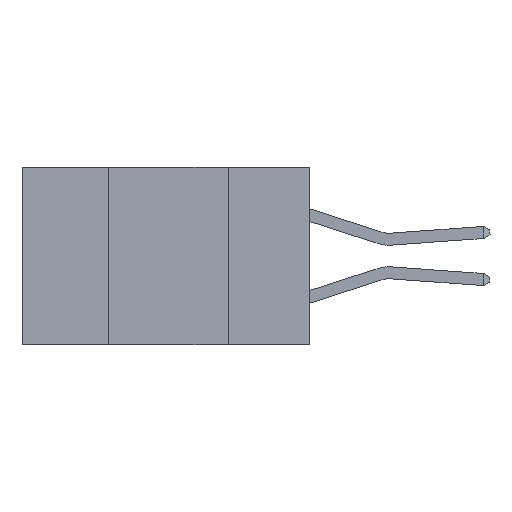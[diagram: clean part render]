
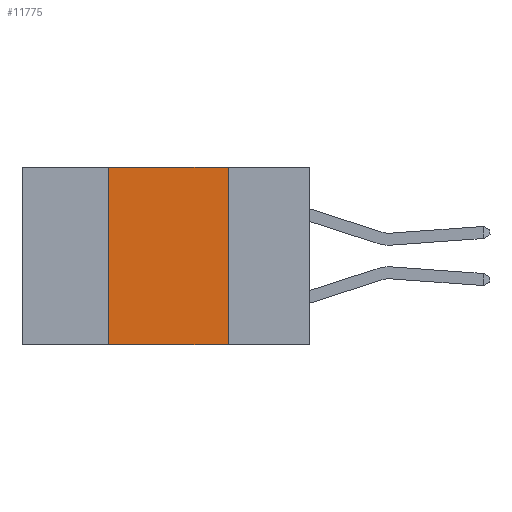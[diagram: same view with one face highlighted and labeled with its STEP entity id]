
A CAD part, left-side view. The second image highlights one B-rep face of the part: STEP entity #11775.
In plain terms, the highlighted planar face has unit normal (-1, 0, 0).
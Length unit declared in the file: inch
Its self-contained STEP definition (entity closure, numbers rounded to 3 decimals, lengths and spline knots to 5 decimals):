
#38 = DIRECTION ( 'NONE',  ( 1., 0., 0. ) ) ;
#1199 = VECTOR ( 'NONE', #7172, 39.37008 ) ;
#1206 = VECTOR ( 'NONE', #1459, 39.37008 ) ;
#1294 = CARTESIAN_POINT ( 'NONE',  ( 0., 0.42, -0.37 ) ) ;
#1459 = DIRECTION ( 'NONE',  ( 0., -1., 0. ) ) ;
#2336 = CARTESIAN_POINT ( 'NONE',  ( 0., 0.17, 0. ) ) ;
#2898 = DIRECTION ( 'NONE',  ( 0., -1., 0. ) ) ;
#3753 = VERTEX_POINT ( 'NONE', #1294 ) ;
#4322 = VERTEX_POINT ( 'NONE', #10105 ) ;
#4729 = LINE ( 'NONE', #11381, #13402 ) ;
#5004 = DIRECTION ( 'NONE',  ( 0., 0., 1. ) ) ;
#5366 = ORIENTED_EDGE ( 'NONE', *, *, #13936, .T. ) ;
#6146 = CARTESIAN_POINT ( 'NONE',  ( 0., 0.42, 0. ) ) ;
#6236 = ORIENTED_EDGE ( 'NONE', *, *, #10648, .F. ) ;
#6549 = FACE_OUTER_BOUND ( 'NONE', #13334, .T. ) ;
#6702 = VECTOR ( 'NONE', #5004, 39.37008 ) ;
#7078 = LINE ( 'NONE', #13237, #6702 ) ;
#7113 = VERTEX_POINT ( 'NONE', #12427 ) ;
#7172 = DIRECTION ( 'NONE',  ( 0., 0., -1. ) ) ;
#7542 = ORIENTED_EDGE ( 'NONE', *, *, #14920, .F. ) ;
#7677 = LINE ( 'NONE', #2336, #1199 ) ;
#8503 = CARTESIAN_POINT ( 'NONE',  ( 0., 0.6, 0. ) ) ;
#8557 = DIRECTION ( 'NONE',  ( 0., 0., -1. ) ) ;
#8748 = CARTESIAN_POINT ( 'NONE',  ( 0., 0.6, -0.37 ) ) ;
#8901 = VERTEX_POINT ( 'NONE', #6146 ) ;
#10105 = CARTESIAN_POINT ( 'NONE',  ( 0., 0.17, -0.37 ) ) ;
#10168 = LINE ( 'NONE', #8748, #1206 ) ;
#10648 = EDGE_CURVE ( 'NONE', #8901, #7113, #4729, .T. ) ;
#11381 = CARTESIAN_POINT ( 'NONE',  ( 0., 0.6, 0. ) ) ;
#11545 = ORIENTED_EDGE ( 'NONE', *, *, #11716, .F. ) ;
#11707 = AXIS2_PLACEMENT_3D ( 'NONE', #8503, #38, #8557 ) ;
#11716 = EDGE_CURVE ( 'NONE', #7113, #4322, #7677, .T. ) ;
#11775 = ADVANCED_FACE ( 'NONE', ( #6549 ), #13207, .F. ) ;
#12427 = CARTESIAN_POINT ( 'NONE',  ( 0., 0.17, 0. ) ) ;
#13207 = PLANE ( 'NONE',  #11707 ) ;
#13237 = CARTESIAN_POINT ( 'NONE',  ( 0., 0.42, 0. ) ) ;
#13334 = EDGE_LOOP ( 'NONE', ( #11545, #6236, #7542, #5366 ) ) ;
#13402 = VECTOR ( 'NONE', #2898, 39.37008 ) ;
#13936 = EDGE_CURVE ( 'NONE', #3753, #4322, #10168, .T. ) ;
#14920 = EDGE_CURVE ( 'NONE', #3753, #8901, #7078, .T. ) ;
